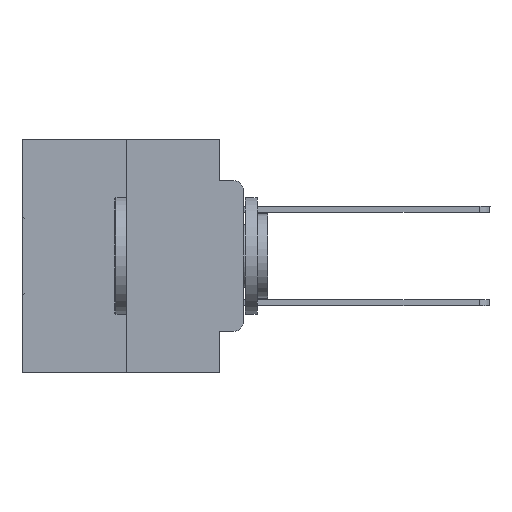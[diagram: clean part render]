
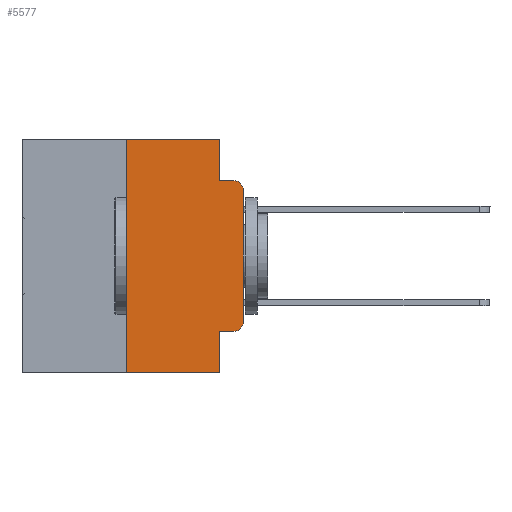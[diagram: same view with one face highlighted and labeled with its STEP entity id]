
A CAD part, left-side view. The second image highlights one B-rep face of the part: STEP entity #5577.
In plain terms, the highlighted planar face has unit normal (-1, 0, 0).
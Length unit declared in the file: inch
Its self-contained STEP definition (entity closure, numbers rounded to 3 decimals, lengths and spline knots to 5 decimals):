
#482 = CARTESIAN_POINT ( 'NONE',  ( 0., 0.25, -0.5 ) ) ;
#1313 = CARTESIAN_POINT ( 'NONE',  ( 0., 0.473, 0. ) ) ;
#1647 = LINE ( 'NONE', #11069, #27686 ) ;
#1862 = LINE ( 'NONE', #25124, #27904 ) ;
#2401 = VECTOR ( 'NONE', #20918, 39.37008 ) ;
#2783 = ORIENTED_EDGE ( 'NONE', *, *, #16220, .T. ) ;
#3421 = VECTOR ( 'NONE', #13824, 39.37008 ) ;
#4782 = ORIENTED_EDGE ( 'NONE', *, *, #16692, .F. ) ;
#4898 = EDGE_CURVE ( 'NONE', #29398, #7978, #23786, .T. ) ;
#5069 = CARTESIAN_POINT ( 'NONE',  ( 0., 0.02, -0.1085 ) ) ;
#5251 = AXIS2_PLACEMENT_3D ( 'NONE', #1313, #11563, #29113 ) ;
#5577 = ADVANCED_FACE ( 'NONE', ( #24922 ), #21535, .F. ) ;
#5787 = CARTESIAN_POINT ( 'NONE',  ( 0., 0.473, 0. ) ) ;
#6234 = EDGE_CURVE ( 'NONE', #14144, #17152, #23521, .T. ) ;
#6374 = CARTESIAN_POINT ( 'NONE',  ( 0., 0.051, -0.4115 ) ) ;
#6402 = ORIENTED_EDGE ( 'NONE', *, *, #30350, .F. ) ;
#6447 = DIRECTION ( 'NONE',  ( 0., 0., 1. ) ) ;
#6574 = LINE ( 'NONE', #7231, #7352 ) ;
#7231 = CARTESIAN_POINT ( 'NONE',  ( 0., 0.473, -0.5 ) ) ;
#7352 = VECTOR ( 'NONE', #14707, 39.37008 ) ;
#7488 = CARTESIAN_POINT ( 'NONE',  ( 0., 0.051, -0.5 ) ) ;
#7612 = DIRECTION ( 'NONE',  ( 0., 0., -1. ) ) ;
#7645 = VECTOR ( 'NONE', #6447, 39.37008 ) ;
#7966 = ORIENTED_EDGE ( 'NONE', *, *, #25175, .T. ) ;
#7978 = VERTEX_POINT ( 'NONE', #21053 ) ;
#8249 = EDGE_CURVE ( 'NONE', #9168, #17152, #6574, .T. ) ;
#9168 = VERTEX_POINT ( 'NONE', #482 ) ;
#9368 = VERTEX_POINT ( 'NONE', #26877 ) ;
#9747 = EDGE_CURVE ( 'NONE', #9368, #28453, #15884, .T. ) ;
#10080 = DIRECTION ( 'NONE',  ( 0., -1., 0. ) ) ;
#10330 = DIRECTION ( 'NONE',  ( 0., 0., 1. ) ) ;
#11069 = CARTESIAN_POINT ( 'NONE',  ( 0., 0.051, 0. ) ) ;
#11522 = CARTESIAN_POINT ( 'NONE',  ( 0., 0.051, 0. ) ) ;
#11563 = DIRECTION ( 'NONE',  ( 1., 0., 0. ) ) ;
#12210 = AXIS2_PLACEMENT_3D ( 'NONE', #5069, #22650, #7612 ) ;
#13824 = DIRECTION ( 'NONE',  ( 0., 0., -1. ) ) ;
#14144 = VERTEX_POINT ( 'NONE', #6374 ) ;
#14308 = LINE ( 'NONE', #15855, #15085 ) ;
#14707 = DIRECTION ( 'NONE',  ( 0., -1., 0. ) ) ;
#14824 = CARTESIAN_POINT ( 'NONE',  ( 0., 0.02, -0.3915 ) ) ;
#15085 = VECTOR ( 'NONE', #28366, 39.37008 ) ;
#15855 = CARTESIAN_POINT ( 'NONE',  ( 0., 0.051, -0.0885 ) ) ;
#15884 = LINE ( 'NONE', #5787, #2401 ) ;
#16114 = DIRECTION ( 'NONE',  ( 0., 0., -1. ) ) ;
#16220 = EDGE_CURVE ( 'NONE', #32340, #29398, #22566, .T. ) ;
#16250 = ORIENTED_EDGE ( 'NONE', *, *, #4898, .T. ) ;
#16336 = CARTESIAN_POINT ( 'NONE',  ( 0., 0.051, 0. ) ) ;
#16692 = EDGE_CURVE ( 'NONE', #18537, #7978, #14308, .T. ) ;
#17152 = VERTEX_POINT ( 'NONE', #7488 ) ;
#17302 = DIRECTION ( 'NONE',  ( 0., 0., -1. ) ) ;
#18537 = VERTEX_POINT ( 'NONE', #31936 ) ;
#19067 = CARTESIAN_POINT ( 'NONE',  ( 0., 0.02, -0.4115 ) ) ;
#19877 = AXIS2_PLACEMENT_3D ( 'NONE', #14824, #32231, #17302 ) ;
#20828 = EDGE_CURVE ( 'NONE', #30138, #32340, #21515, .T. ) ;
#20918 = DIRECTION ( 'NONE',  ( 0., -1., 0. ) ) ;
#21053 = CARTESIAN_POINT ( 'NONE',  ( 0., 0.02, -0.0885 ) ) ;
#21359 = CARTESIAN_POINT ( 'NONE',  ( 0., 0., 0. ) ) ;
#21515 = CIRCLE ( 'NONE', #19877, 0.02 ) ;
#21535 = PLANE ( 'NONE',  #5251 ) ;
#21892 = CARTESIAN_POINT ( 'NONE',  ( 0., 0., -0.3915 ) ) ;
#22078 = VECTOR ( 'NONE', #10330, 39.37008 ) ;
#22099 = ORIENTED_EDGE ( 'NONE', *, *, #20828, .T. ) ;
#22566 = LINE ( 'NONE', #21359, #7645 ) ;
#22650 = DIRECTION ( 'NONE',  ( -1., 0., 0. ) ) ;
#22816 = CARTESIAN_POINT ( 'NONE',  ( 0., 0.25, 0. ) ) ;
#23521 = LINE ( 'NONE', #16336, #3421 ) ;
#23786 = CIRCLE ( 'NONE', #12210, 0.02 ) ;
#24852 = ORIENTED_EDGE ( 'NONE', *, *, #28914, .F. ) ;
#24922 = FACE_OUTER_BOUND ( 'NONE', #30706, .T. ) ;
#25124 = CARTESIAN_POINT ( 'NONE',  ( 0., 0.051, -0.4115 ) ) ;
#25175 = EDGE_CURVE ( 'NONE', #14144, #30138, #1862, .T. ) ;
#26418 = ORIENTED_EDGE ( 'NONE', *, *, #8249, .T. ) ;
#26877 = CARTESIAN_POINT ( 'NONE',  ( 0., 0.25, 0. ) ) ;
#27195 = ORIENTED_EDGE ( 'NONE', *, *, #6234, .F. ) ;
#27686 = VECTOR ( 'NONE', #16114, 39.37008 ) ;
#27904 = VECTOR ( 'NONE', #10080, 39.37008 ) ;
#28366 = DIRECTION ( 'NONE',  ( 0., -1., 0. ) ) ;
#28453 = VERTEX_POINT ( 'NONE', #11522 ) ;
#28914 = EDGE_CURVE ( 'NONE', #28453, #18537, #1647, .T. ) ;
#29113 = DIRECTION ( 'NONE',  ( 0., 0., -1. ) ) ;
#29398 = VERTEX_POINT ( 'NONE', #30922 ) ;
#29538 = LINE ( 'NONE', #22816, #22078 ) ;
#30138 = VERTEX_POINT ( 'NONE', #19067 ) ;
#30350 = EDGE_CURVE ( 'NONE', #9168, #9368, #29538, .T. ) ;
#30706 = EDGE_LOOP ( 'NONE', ( #2783, #16250, #4782, #24852, #32178, #6402, #26418, #27195, #7966, #22099 ) ) ;
#30922 = CARTESIAN_POINT ( 'NONE',  ( 0., 0., -0.1085 ) ) ;
#31936 = CARTESIAN_POINT ( 'NONE',  ( 0., 0.051, -0.0885 ) ) ;
#32178 = ORIENTED_EDGE ( 'NONE', *, *, #9747, .F. ) ;
#32231 = DIRECTION ( 'NONE',  ( -1., 0., 0. ) ) ;
#32340 = VERTEX_POINT ( 'NONE', #21892 ) ;
